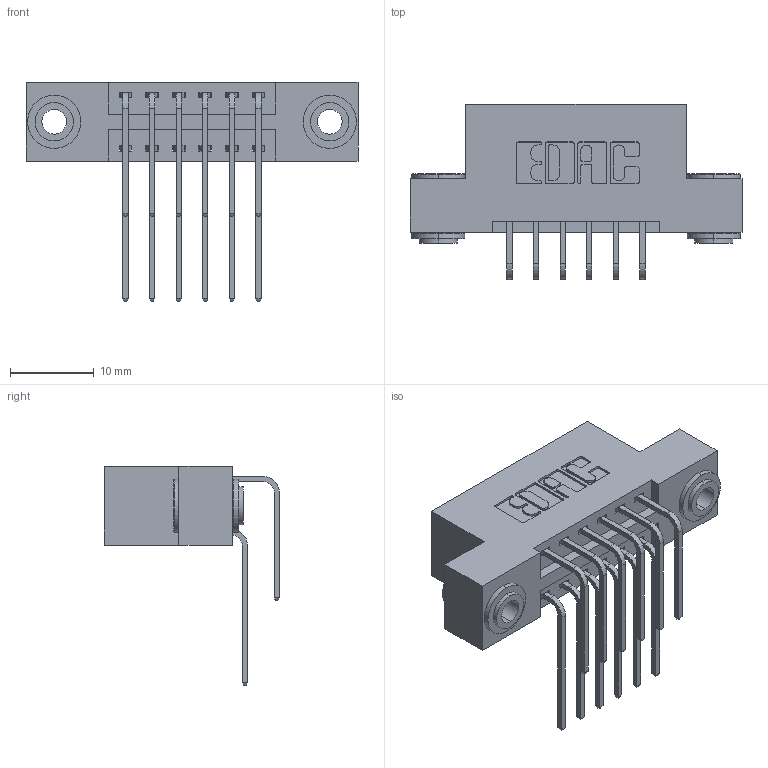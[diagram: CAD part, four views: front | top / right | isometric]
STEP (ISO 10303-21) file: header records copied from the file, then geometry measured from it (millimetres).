
FILE_DESCRIPTION (( 'STEP AP203' ), '1' );
FILE_NAME ('396-012-559-203.STEP', '2018-08-31T07:23:20', ( '' ), ( '' ), 'SwSTEP 2.0', 'SolidWorks 2016', '' );
FILE_SCHEMA (( 'CONFIG_CONTROL_DESIGN' ));
Length unit declared in the file: inch
Products named in the file (5): 396-012-559-203; 346 Part_Flush Mounting Lugs - 0.156 Dia-TH; 345-292-001_558 559 Tail - 1; 345-292-001_559 Tail - 2; 345-250-002_345-250-002-102
Assembly tree (15 placements, depth 2):
  396-012-559-203
    346 Part_Flush Mounting Lugs - 0.156 Dia-TH
    345-292-001_558 559 Tail - 1  x6
    345-292-001_559 Tail - 2  x6
    345-250-002_345-250-002-102  x2
Bounding box: 39.62 x 20.89 x 26.16 mm (x, y, z)
Volume: 3672.8 mm3; surface area: 5029 mm2
Topology: 15 solids, 15 shells, 808 faces, 2337 edges, 1538 vertices
Faces by surface type: plane 530, cylinder 270, cone 8
Entity records: 11196 total; most frequent: CARTESIAN_POINT 1922, ORIENTED_EDGE 1798, DIRECTION 1749, EDGE_CURVE 899, VECTOR 679, LINE 679, VERTEX_POINT 594, AXIS2_PLACEMENT_3D 535
